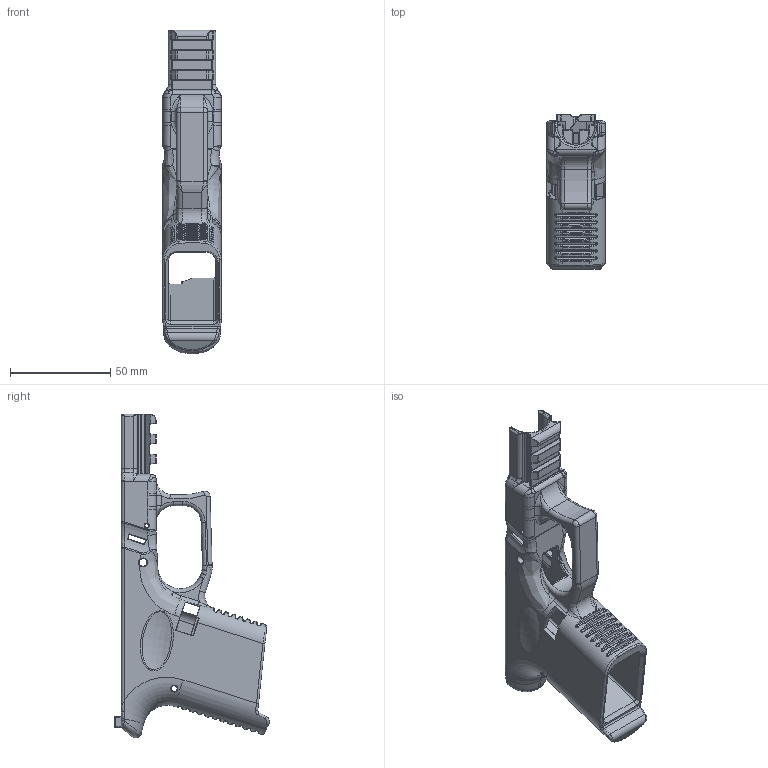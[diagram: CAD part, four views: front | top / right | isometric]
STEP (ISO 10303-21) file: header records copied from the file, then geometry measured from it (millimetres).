
FILE_DESCRIPTION(/* description */ (''),/* implementation_level */ '2;1');
FILE_NAME(/* name */ 'G26 P80.step',/* time_stamp */ '2019-11-24T19:36:38-05:00',/* author */ (''),/* organization */ (''),/* preprocessor_version */ 'ST-DEVELOPER v18',/* originating_system */ 'Autodesk Translation Framework v8.12.0.6',/* authorisation */ '');
FILE_SCHEMA (('AUTOMOTIVE_DESIGN { 1 0 10303 214 3 1 1 }'));
Length unit declared in the file: millimetre
Products named in the file (1): G26 P80
Bounding box: 29.21 x 77.09 x 161.39 mm (x, y, z)
Volume: 68916.3 mm3; surface area: 36644.7 mm2
Topology: 1 solids, 1 shells, 1554 faces, 3715 edges, 2067 vertices
Faces by surface type: bspline 602, cylinder 481, plane 237, torus 162, sphere 58, cone 14
Full cylindrical faces by diameter (mm): 2 x4, 2.997 x2, 3.962 x2, 4 x1
Entity records: 72364 total; most frequent: CARTESIAN_POINT 39295, ORIENTED_EDGE 7262, DIRECTION 6449, EDGE_CURVE 3631, AXIS2_PLACEMENT_3D 2677, VERTEX_POINT 2067, EDGE_LOOP 1568, FACE_OUTER_BOUND 1552
